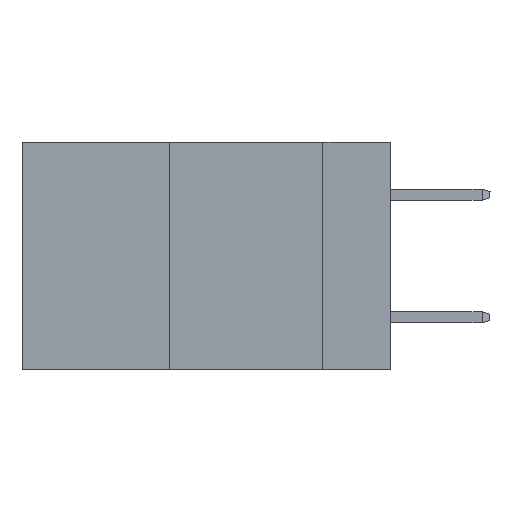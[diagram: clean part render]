
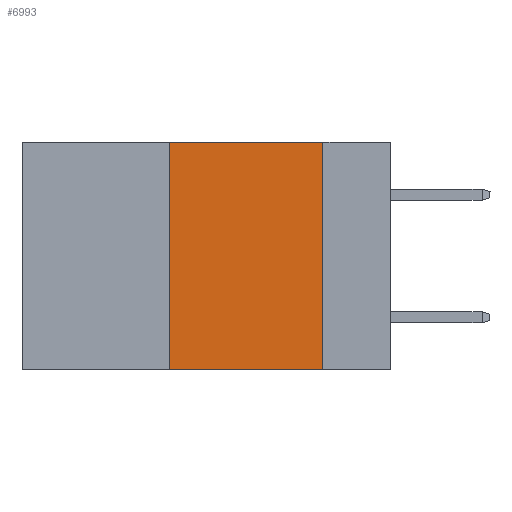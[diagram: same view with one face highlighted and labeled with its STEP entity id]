
A CAD part, left-side view. The second image highlights one B-rep face of the part: STEP entity #6993.
In plain terms, the highlighted planar face has unit normal (-1, 0, 0).
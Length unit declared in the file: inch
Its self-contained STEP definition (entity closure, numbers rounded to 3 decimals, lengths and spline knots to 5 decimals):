
#417 = CARTESIAN_POINT ( 'NONE',  ( 0., 0.11, 0. ) ) ;
#2836 = VECTOR ( 'NONE', #14691, 39.37008 ) ;
#3229 = DIRECTION ( 'NONE',  ( 0., 0., 1. ) ) ;
#3306 = PLANE ( 'NONE',  #14769 ) ;
#3313 = VECTOR ( 'NONE', #10198, 39.37008 ) ;
#3350 = CARTESIAN_POINT ( 'NONE',  ( 0., 0.6, 0. ) ) ;
#3725 = DIRECTION ( 'NONE',  ( 0., 0., -1. ) ) ;
#4044 = CARTESIAN_POINT ( 'NONE',  ( 0., 0.36, 0. ) ) ;
#4281 = EDGE_CURVE ( 'NONE', #10625, #8557, #5371, .T. ) ;
#4561 = DIRECTION ( 'NONE',  ( 0., 0., -1. ) ) ;
#4745 = VERTEX_POINT ( 'NONE', #10646 ) ;
#5371 = LINE ( 'NONE', #3350, #3313 ) ;
#5712 = DIRECTION ( 'NONE',  ( 1., 0., 0. ) ) ;
#5881 = ORIENTED_EDGE ( 'NONE', *, *, #4281, .F. ) ;
#6710 = EDGE_CURVE ( 'NONE', #14867, #4745, #10255, .T. ) ;
#6838 = VECTOR ( 'NONE', #3229, 39.37008 ) ;
#6878 = FACE_OUTER_BOUND ( 'NONE', #9920, .T. ) ;
#6993 = ADVANCED_FACE ( 'NONE', ( #6878 ), #3306, .F. ) ;
#7412 = ORIENTED_EDGE ( 'NONE', *, *, #9873, .F. ) ;
#8300 = EDGE_CURVE ( 'NONE', #14867, #10625, #12743, .T. ) ;
#8557 = VERTEX_POINT ( 'NONE', #417 ) ;
#9873 = EDGE_CURVE ( 'NONE', #8557, #4745, #12155, .T. ) ;
#9920 = EDGE_LOOP ( 'NONE', ( #7412, #5881, #15115, #14743 ) ) ;
#10198 = DIRECTION ( 'NONE',  ( 0., -1., 0. ) ) ;
#10255 = LINE ( 'NONE', #12620, #2836 ) ;
#10466 = CARTESIAN_POINT ( 'NONE',  ( 0., 0.36, 0. ) ) ;
#10625 = VERTEX_POINT ( 'NONE', #4044 ) ;
#10646 = CARTESIAN_POINT ( 'NONE',  ( 0., 0.11, -0.37 ) ) ;
#10791 = CARTESIAN_POINT ( 'NONE',  ( 0., 0.36, -0.37 ) ) ;
#11680 = CARTESIAN_POINT ( 'NONE',  ( 0., 0.6, 0. ) ) ;
#12155 = LINE ( 'NONE', #13662, #14466 ) ;
#12620 = CARTESIAN_POINT ( 'NONE',  ( 0., 0.6, -0.37 ) ) ;
#12743 = LINE ( 'NONE', #10466, #6838 ) ;
#13662 = CARTESIAN_POINT ( 'NONE',  ( 0., 0.11, 0. ) ) ;
#14466 = VECTOR ( 'NONE', #3725, 39.37008 ) ;
#14691 = DIRECTION ( 'NONE',  ( 0., -1., 0. ) ) ;
#14743 = ORIENTED_EDGE ( 'NONE', *, *, #6710, .T. ) ;
#14769 = AXIS2_PLACEMENT_3D ( 'NONE', #11680, #5712, #4561 ) ;
#14867 = VERTEX_POINT ( 'NONE', #10791 ) ;
#15115 = ORIENTED_EDGE ( 'NONE', *, *, #8300, .F. ) ;
